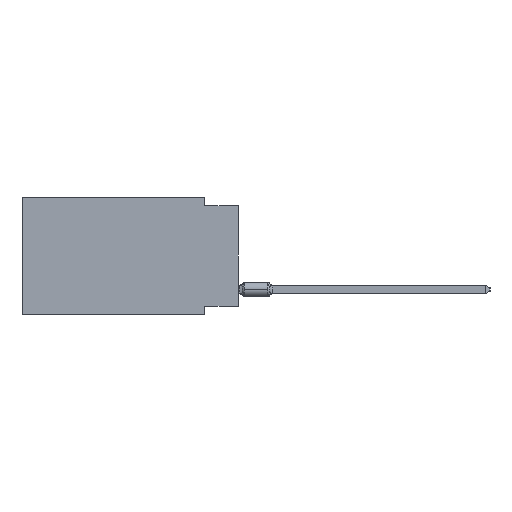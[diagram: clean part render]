
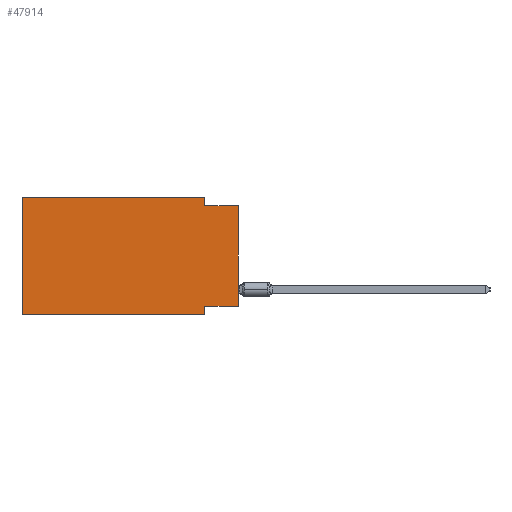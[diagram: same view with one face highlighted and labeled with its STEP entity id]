
A CAD part, left-side view. The second image highlights one B-rep face of the part: STEP entity #47914.
In plain terms, the highlighted planar face has unit normal (-1, 0, 0).
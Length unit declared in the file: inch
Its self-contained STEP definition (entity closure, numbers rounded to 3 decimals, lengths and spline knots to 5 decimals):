
#670 = EDGE_LOOP ( 'NONE', ( #20866, #24710, #6028, #42135, #26074, #44034, #19064, #26886 ) ) ;
#2358 = CARTESIAN_POINT ( 'NONE',  ( 0., 0.645, -0.35 ) ) ;
#2986 = CARTESIAN_POINT ( 'NONE',  ( 0., 0.645, -0.35 ) ) ;
#3381 = CARTESIAN_POINT ( 'NONE',  ( 0., 0.645, 0. ) ) ;
#4899 = VERTEX_POINT ( 'NONE', #40026 ) ;
#5714 = CARTESIAN_POINT ( 'NONE',  ( 0., 0.1, -0.35 ) ) ;
#6028 = ORIENTED_EDGE ( 'NONE', *, *, #41625, .F. ) ;
#6045 = EDGE_CURVE ( 'NONE', #48439, #15661, #20215, .T. ) ;
#6236 = EDGE_CURVE ( 'NONE', #37358, #4899, #23295, .T. ) ;
#7071 = VECTOR ( 'NONE', #12546, 39.37008 ) ;
#10218 = DIRECTION ( 'NONE',  ( 0., -1., 0. ) ) ;
#12282 = LINE ( 'NONE', #36276, #7071 ) ;
#12546 = DIRECTION ( 'NONE',  ( 0., 0., 1. ) ) ;
#14558 = CARTESIAN_POINT ( 'NONE',  ( 0., 0.1, 0. ) ) ;
#15648 = EDGE_CURVE ( 'NONE', #48925, #48252, #18555, .T. ) ;
#15661 = VERTEX_POINT ( 'NONE', #30685 ) ;
#16111 = CARTESIAN_POINT ( 'NONE',  ( 0., 0., -0.325 ) ) ;
#18555 = LINE ( 'NONE', #2986, #44130 ) ;
#19064 = ORIENTED_EDGE ( 'NONE', *, *, #39637, .F. ) ;
#19490 = DIRECTION ( 'NONE',  ( 0., 0., -1. ) ) ;
#20215 = LINE ( 'NONE', #32080, #30154 ) ;
#20239 = VECTOR ( 'NONE', #26213, 39.37008 ) ;
#20866 = ORIENTED_EDGE ( 'NONE', *, *, #6045, .T. ) ;
#22906 = DIRECTION ( 'NONE',  ( 1., 0., 0. ) ) ;
#23295 = LINE ( 'NONE', #30964, #20239 ) ;
#24154 = VERTEX_POINT ( 'NONE', #46582 ) ;
#24710 = ORIENTED_EDGE ( 'NONE', *, *, #45044, .F. ) ;
#25392 = EDGE_CURVE ( 'NONE', #48439, #24154, #43529, .T. ) ;
#26074 = ORIENTED_EDGE ( 'NONE', *, *, #30962, .F. ) ;
#26213 = DIRECTION ( 'NONE',  ( 0., -1., 0. ) ) ;
#26744 = CARTESIAN_POINT ( 'NONE',  ( 0., 0.1, -0.35 ) ) ;
#26886 = ORIENTED_EDGE ( 'NONE', *, *, #25392, .F. ) ;
#27700 = VECTOR ( 'NONE', #10218, 39.37008 ) ;
#30154 = VECTOR ( 'NONE', #48140, 39.37008 ) ;
#30283 = LINE ( 'NONE', #46328, #27700 ) ;
#30641 = DIRECTION ( 'NONE',  ( 0., 0., -1. ) ) ;
#30685 = CARTESIAN_POINT ( 'NONE',  ( 0., 0., -0.025 ) ) ;
#30962 = EDGE_CURVE ( 'NONE', #48925, #37358, #12282, .T. ) ;
#30964 = CARTESIAN_POINT ( 'NONE',  ( 0., 0.645, 0. ) ) ;
#32080 = CARTESIAN_POINT ( 'NONE',  ( 0., 0., 0. ) ) ;
#34231 = LINE ( 'NONE', #5714, #40333 ) ;
#34645 = DIRECTION ( 'NONE',  ( 0., -1., 0. ) ) ;
#36276 = CARTESIAN_POINT ( 'NONE',  ( 0., 0.645, 0. ) ) ;
#36588 = AXIS2_PLACEMENT_3D ( 'NONE', #3381, #22906, #19490 ) ;
#37358 = VERTEX_POINT ( 'NONE', #38302 ) ;
#38302 = CARTESIAN_POINT ( 'NONE',  ( 0., 0.645, 0. ) ) ;
#38864 = CARTESIAN_POINT ( 'NONE',  ( 0., 0.1, -0.025 ) ) ;
#39581 = VECTOR ( 'NONE', #39817, 39.37008 ) ;
#39637 = EDGE_CURVE ( 'NONE', #24154, #48252, #34231, .T. ) ;
#39817 = DIRECTION ( 'NONE',  ( 0., 1., 0. ) ) ;
#40026 = CARTESIAN_POINT ( 'NONE',  ( 0., 0.1, 0. ) ) ;
#40333 = VECTOR ( 'NONE', #50012, 39.37008 ) ;
#41625 = EDGE_CURVE ( 'NONE', #4899, #42268, #50657, .T. ) ;
#42135 = ORIENTED_EDGE ( 'NONE', *, *, #6236, .F. ) ;
#42268 = VERTEX_POINT ( 'NONE', #38864 ) ;
#43529 = LINE ( 'NONE', #16111, #39581 ) ;
#44034 = ORIENTED_EDGE ( 'NONE', *, *, #15648, .T. ) ;
#44130 = VECTOR ( 'NONE', #34645, 39.37008 ) ;
#45044 = EDGE_CURVE ( 'NONE', #42268, #15661, #30283, .T. ) ;
#45645 = CARTESIAN_POINT ( 'NONE',  ( 0., 0., -0.325 ) ) ;
#46328 = CARTESIAN_POINT ( 'NONE',  ( 0., 0., -0.025 ) ) ;
#46582 = CARTESIAN_POINT ( 'NONE',  ( 0., 0.1, -0.325 ) ) ;
#46779 = VECTOR ( 'NONE', #30641, 39.37008 ) ;
#46894 = PLANE ( 'NONE',  #36588 ) ;
#47161 = FACE_OUTER_BOUND ( 'NONE', #670, .T. ) ;
#47914 = ADVANCED_FACE ( 'NONE', ( #47161 ), #46894, .F. ) ;
#48140 = DIRECTION ( 'NONE',  ( 0., 0., 1. ) ) ;
#48252 = VERTEX_POINT ( 'NONE', #26744 ) ;
#48439 = VERTEX_POINT ( 'NONE', #45645 ) ;
#48925 = VERTEX_POINT ( 'NONE', #2358 ) ;
#50012 = DIRECTION ( 'NONE',  ( 0., 0., -1. ) ) ;
#50657 = LINE ( 'NONE', #14558, #46779 ) ;
